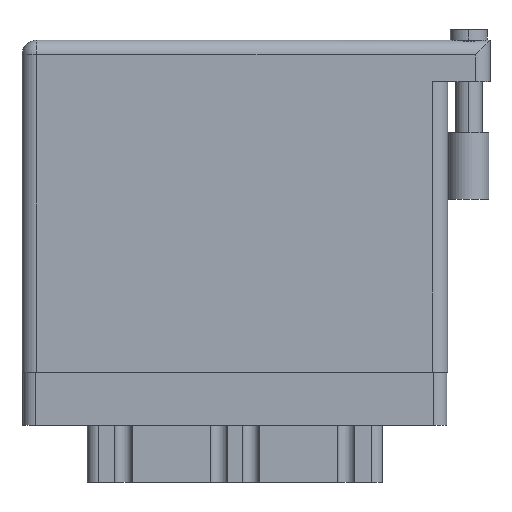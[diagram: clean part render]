
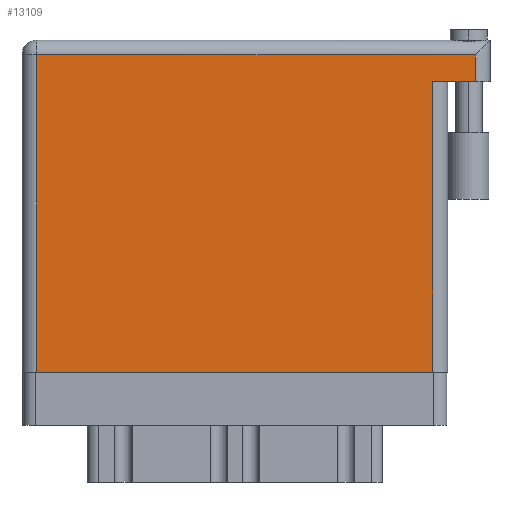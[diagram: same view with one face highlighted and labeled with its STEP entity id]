
A CAD part, front view. The second image highlights one B-rep face of the part: STEP entity #13109.
In plain terms, the highlighted face is planar.
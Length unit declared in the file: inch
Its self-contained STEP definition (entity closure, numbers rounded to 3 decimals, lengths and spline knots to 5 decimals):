
#274 = FACE_OUTER_BOUND ( 'NONE', #29857, .T. ) ;
#2048 = VERTEX_POINT ( 'NONE', #21868 ) ;
#3267 = EDGE_CURVE ( 'NONE', #3848, #3992, #22328, .T. ) ;
#3691 = DIRECTION ( 'NONE',  ( 0., 1., 0. ) ) ;
#3799 = DIRECTION ( 'NONE',  ( 0., 1., 0. ) ) ;
#3848 = VERTEX_POINT ( 'NONE', #34182 ) ;
#3930 = CARTESIAN_POINT ( 'NONE',  ( 0.07, 0., 0. ) ) ;
#3992 = VERTEX_POINT ( 'NONE', #4917 ) ;
#4384 = VECTOR ( 'NONE', #8892, 39.37008 ) ;
#4917 = CARTESIAN_POINT ( 'NONE',  ( 1.938, 1.369, 0. ) ) ;
#5230 = LINE ( 'NONE', #13812, #37483 ) ;
#6339 = ORIENTED_EDGE ( 'NONE', *, *, #37158, .T. ) ;
#6463 = VECTOR ( 'NONE', #3691, 39.37008 ) ;
#7156 = LINE ( 'NONE', #33478, #31353 ) ;
#8892 = DIRECTION ( 'NONE',  ( 0., -1., 0. ) ) ;
#9146 = VERTEX_POINT ( 'NONE', #27640 ) ;
#9432 = PLANE ( 'NONE',  #37176 ) ;
#10117 = CARTESIAN_POINT ( 'NONE',  ( 2.138, 1.566, 0. ) ) ;
#10377 = EDGE_CURVE ( 'NONE', #21725, #9146, #15775, .T. ) ;
#10524 = ORIENTED_EDGE ( 'NONE', *, *, #3267, .T. ) ;
#11639 = DIRECTION ( 'NONE',  ( -1., 0., 0. ) ) ;
#12155 = CARTESIAN_POINT ( 'NONE',  ( 0., 1.566, 0. ) ) ;
#12803 = DIRECTION ( 'NONE',  ( 1., 0., 0. ) ) ;
#13109 = ADVANCED_FACE ( 'NONE', ( #274 ), #9432, .F. ) ;
#13812 = CARTESIAN_POINT ( 'NONE',  ( 2.208, 1.369, 0. ) ) ;
#14760 = LINE ( 'NONE', #20019, #37675 ) ;
#14857 = VERTEX_POINT ( 'NONE', #3930 ) ;
#15697 = EDGE_CURVE ( 'NONE', #21725, #3992, #5230, .T. ) ;
#15775 = LINE ( 'NONE', #10117, #6463 ) ;
#15900 = ORIENTED_EDGE ( 'NONE', *, *, #20514, .T. ) ;
#17116 = DIRECTION ( 'NONE',  ( -1., 0., 0. ) ) ;
#17292 = LINE ( 'NONE', #29169, #4384 ) ;
#17895 = ORIENTED_EDGE ( 'NONE', *, *, #10377, .T. ) ;
#18592 = DIRECTION ( 'NONE',  ( 0., 0., -1. ) ) ;
#20019 = CARTESIAN_POINT ( 'NONE',  ( 0., 1.496, 0. ) ) ;
#20514 = EDGE_CURVE ( 'NONE', #9146, #2048, #14760, .T. ) ;
#20950 = CARTESIAN_POINT ( 'NONE',  ( 2.138, 1.369, 0. ) ) ;
#21725 = VERTEX_POINT ( 'NONE', #20950 ) ;
#21868 = CARTESIAN_POINT ( 'NONE',  ( 0.07, 1.496, 0. ) ) ;
#22328 = LINE ( 'NONE', #25442, #37080 ) ;
#22767 = ORIENTED_EDGE ( 'NONE', *, *, #25087, .T. ) ;
#25087 = EDGE_CURVE ( 'NONE', #2048, #14857, #17292, .T. ) ;
#25251 = ORIENTED_EDGE ( 'NONE', *, *, #15697, .F. ) ;
#25442 = CARTESIAN_POINT ( 'NONE',  ( 1.938, 1.369, 0. ) ) ;
#27640 = CARTESIAN_POINT ( 'NONE',  ( 2.138, 1.496, 0. ) ) ;
#29169 = CARTESIAN_POINT ( 'NONE',  ( 0.07, 0., 0. ) ) ;
#29857 = EDGE_LOOP ( 'NONE', ( #6339, #10524, #25251, #17895, #15900, #22767 ) ) ;
#31353 = VECTOR ( 'NONE', #12803, 39.37008 ) ;
#33478 = CARTESIAN_POINT ( 'NONE',  ( 0., 0., 0. ) ) ;
#34182 = CARTESIAN_POINT ( 'NONE',  ( 1.938, 0., 0. ) ) ;
#36345 = DIRECTION ( 'NONE',  ( -1., 0., 0. ) ) ;
#37080 = VECTOR ( 'NONE', #3799, 39.37008 ) ;
#37158 = EDGE_CURVE ( 'NONE', #14857, #3848, #7156, .T. ) ;
#37176 = AXIS2_PLACEMENT_3D ( 'NONE', #12155, #18592, #36345 ) ;
#37483 = VECTOR ( 'NONE', #17116, 39.37008 ) ;
#37675 = VECTOR ( 'NONE', #11639, 39.37008 ) ;
